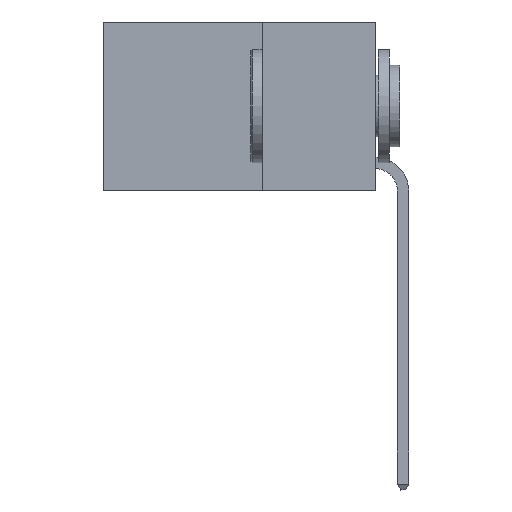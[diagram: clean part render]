
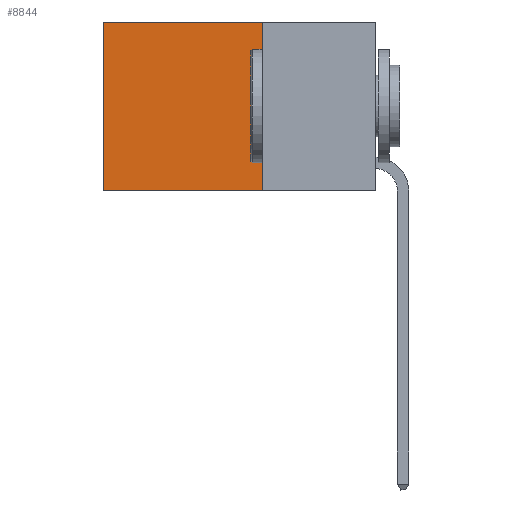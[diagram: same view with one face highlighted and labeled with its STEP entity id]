
A CAD part, left-side view. The second image highlights one B-rep face of the part: STEP entity #8844.
In plain terms, the highlighted planar face has unit normal (-1, 0, 0).
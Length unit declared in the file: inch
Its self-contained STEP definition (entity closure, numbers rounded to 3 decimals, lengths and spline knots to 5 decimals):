
#521 = ORIENTED_EDGE ( 'NONE', *, *, #3631, .F. ) ;
#873 = DIRECTION ( 'NONE',  ( 0., 0., -1. ) ) ;
#1045 = DIRECTION ( 'NONE',  ( 0., 1., 0. ) ) ;
#1157 = CARTESIAN_POINT ( 'NONE',  ( 0.2625, 0.25, 0. ) ) ;
#1732 = CARTESIAN_POINT ( 'NONE',  ( 0.2625, 0.25, 0. ) ) ;
#2193 = DIRECTION ( 'NONE',  ( 0., 1., 0. ) ) ;
#2935 = FACE_OUTER_BOUND ( 'NONE', #5477, .T. ) ;
#3081 = VECTOR ( 'NONE', #1045, 39.37008 ) ;
#3100 = CARTESIAN_POINT ( 'NONE',  ( 0.2625, 0.25, 0. ) ) ;
#3631 = EDGE_CURVE ( 'NONE', #7977, #7381, #3883, .T. ) ;
#3883 = LINE ( 'NONE', #9900, #5960 ) ;
#4934 = CARTESIAN_POINT ( 'NONE',  ( 0.2625, 0.6, 0. ) ) ;
#5046 = ORIENTED_EDGE ( 'NONE', *, *, #7709, .T. ) ;
#5439 = LINE ( 'NONE', #1157, #3081 ) ;
#5477 = EDGE_LOOP ( 'NONE', ( #5046, #521, #10306, #9418 ) ) ;
#5806 = EDGE_CURVE ( 'NONE', #6110, #7832, #5439, .T. ) ;
#5960 = VECTOR ( 'NONE', #2193, 39.37008 ) ;
#6110 = VERTEX_POINT ( 'NONE', #1732 ) ;
#6521 = LINE ( 'NONE', #4934, #9112 ) ;
#6684 = AXIS2_PLACEMENT_3D ( 'NONE', #3100, #9974, #10229 ) ;
#7340 = PLANE ( 'NONE',  #6684 ) ;
#7381 = VERTEX_POINT ( 'NONE', #7665 ) ;
#7665 = CARTESIAN_POINT ( 'NONE',  ( 0.2625, 0.6, -0.37 ) ) ;
#7709 = EDGE_CURVE ( 'NONE', #7832, #7381, #6521, .T. ) ;
#7832 = VERTEX_POINT ( 'NONE', #9110 ) ;
#7977 = VERTEX_POINT ( 'NONE', #10005 ) ;
#8844 = ADVANCED_FACE ( 'NONE', ( #2935 ), #7340, .F. ) ;
#9110 = CARTESIAN_POINT ( 'NONE',  ( 0.2625, 0.6, 0. ) ) ;
#9112 = VECTOR ( 'NONE', #10898, 39.37008 ) ;
#9294 = CARTESIAN_POINT ( 'NONE',  ( 0.2625, 0.25, 0. ) ) ;
#9418 = ORIENTED_EDGE ( 'NONE', *, *, #5806, .T. ) ;
#9900 = CARTESIAN_POINT ( 'NONE',  ( 0.2625, 0.25, -0.37 ) ) ;
#9974 = DIRECTION ( 'NONE',  ( 1., 0., 0. ) ) ;
#10005 = CARTESIAN_POINT ( 'NONE',  ( 0.2625, 0.25, -0.37 ) ) ;
#10159 = EDGE_CURVE ( 'NONE', #6110, #7977, #10289, .T. ) ;
#10229 = DIRECTION ( 'NONE',  ( 0., 0., -1. ) ) ;
#10289 = LINE ( 'NONE', #9294, #11066 ) ;
#10306 = ORIENTED_EDGE ( 'NONE', *, *, #10159, .F. ) ;
#10898 = DIRECTION ( 'NONE',  ( 0., 0., -1. ) ) ;
#11066 = VECTOR ( 'NONE', #873, 39.37008 ) ;
